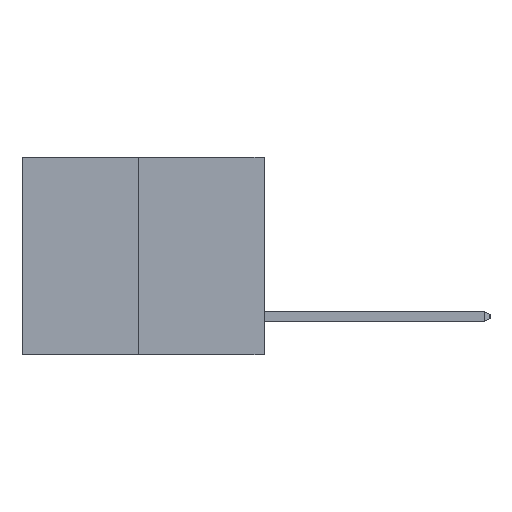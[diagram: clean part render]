
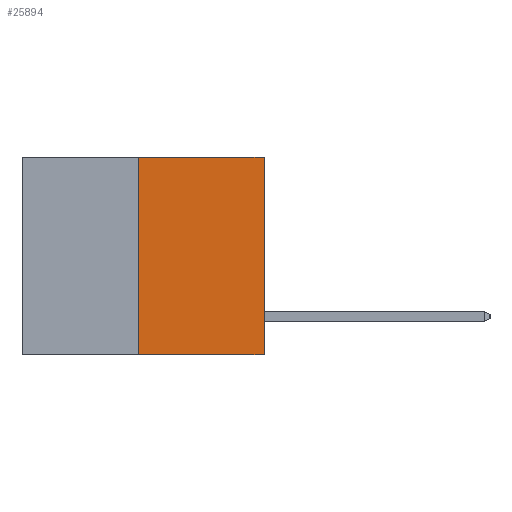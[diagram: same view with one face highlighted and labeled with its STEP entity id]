
A CAD part, left-side view. The second image highlights one B-rep face of the part: STEP entity #25894.
In plain terms, the highlighted planar face has unit normal (-1, 0, 0).
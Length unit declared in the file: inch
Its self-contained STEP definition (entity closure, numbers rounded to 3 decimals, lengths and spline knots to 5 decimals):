
#363 = EDGE_CURVE ( 'NONE', #15989, #3454, #11125, .T. ) ;
#726 = DIRECTION ( 'NONE',  ( 0., -1., 0. ) ) ;
#1678 = DIRECTION ( 'NONE',  ( 1., 0., 0. ) ) ;
#1717 = VERTEX_POINT ( 'NONE', #22267 ) ;
#2130 = CARTESIAN_POINT ( 'NONE',  ( 0., 0.312, 0. ) ) ;
#3026 = VECTOR ( 'NONE', #21756, 39.37008 ) ;
#3163 = AXIS2_PLACEMENT_3D ( 'NONE', #22600, #1678, #16257 ) ;
#3454 = VERTEX_POINT ( 'NONE', #25242 ) ;
#8205 = EDGE_CURVE ( 'NONE', #3454, #1717, #17961, .T. ) ;
#9072 = CARTESIAN_POINT ( 'NONE',  ( 0., 0.6, -0.49 ) ) ;
#9086 = EDGE_CURVE ( 'NONE', #15989, #15437, #14948, .T. ) ;
#9433 = CARTESIAN_POINT ( 'NONE',  ( 0., 0.312, -0.49 ) ) ;
#11125 = LINE ( 'NONE', #9072, #19373 ) ;
#12388 = PLANE ( 'NONE',  #3163 ) ;
#13395 = CARTESIAN_POINT ( 'NONE',  ( 0., 0.6, 0. ) ) ;
#14948 = LINE ( 'NONE', #9433, #3026 ) ;
#15437 = VERTEX_POINT ( 'NONE', #2130 ) ;
#15989 = VERTEX_POINT ( 'NONE', #19896 ) ;
#16198 = FACE_OUTER_BOUND ( 'NONE', #26024, .T. ) ;
#16257 = DIRECTION ( 'NONE',  ( 0., 0., -1. ) ) ;
#16527 = VECTOR ( 'NONE', #726, 39.37008 ) ;
#17961 = LINE ( 'NONE', #18908, #25208 ) ;
#18520 = ORIENTED_EDGE ( 'NONE', *, *, #21314, .F. ) ;
#18908 = CARTESIAN_POINT ( 'NONE',  ( 0., 0., 0. ) ) ;
#19373 = VECTOR ( 'NONE', #25757, 39.37008 ) ;
#19896 = CARTESIAN_POINT ( 'NONE',  ( 0., 0.312, -0.49 ) ) ;
#21314 = EDGE_CURVE ( 'NONE', #15437, #1717, #21454, .T. ) ;
#21454 = LINE ( 'NONE', #13395, #16527 ) ;
#21756 = DIRECTION ( 'NONE',  ( 0., 0., 1. ) ) ;
#22267 = CARTESIAN_POINT ( 'NONE',  ( 0., 0., 0. ) ) ;
#22600 = CARTESIAN_POINT ( 'NONE',  ( 0., 0.6, 0. ) ) ;
#22837 = DIRECTION ( 'NONE',  ( 0., 0., 1. ) ) ;
#23387 = ORIENTED_EDGE ( 'NONE', *, *, #9086, .F. ) ;
#24572 = ORIENTED_EDGE ( 'NONE', *, *, #363, .T. ) ;
#25208 = VECTOR ( 'NONE', #22837, 39.37008 ) ;
#25242 = CARTESIAN_POINT ( 'NONE',  ( 0., 0., -0.49 ) ) ;
#25757 = DIRECTION ( 'NONE',  ( 0., -1., 0. ) ) ;
#25894 = ADVANCED_FACE ( 'NONE', ( #16198 ), #12388, .F. ) ;
#26024 = EDGE_LOOP ( 'NONE', ( #23387, #24572, #27316, #18520 ) ) ;
#27316 = ORIENTED_EDGE ( 'NONE', *, *, #8205, .T. ) ;
